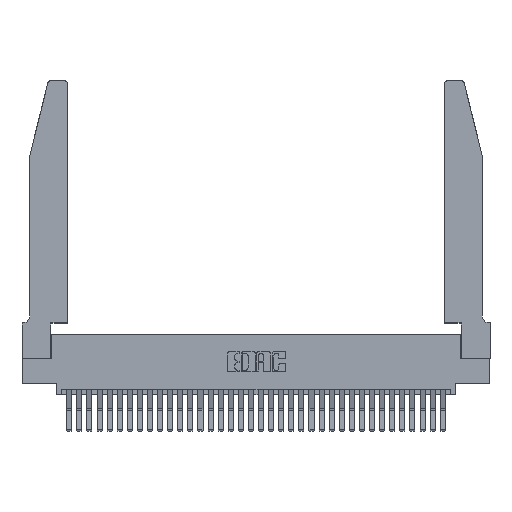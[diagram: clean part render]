
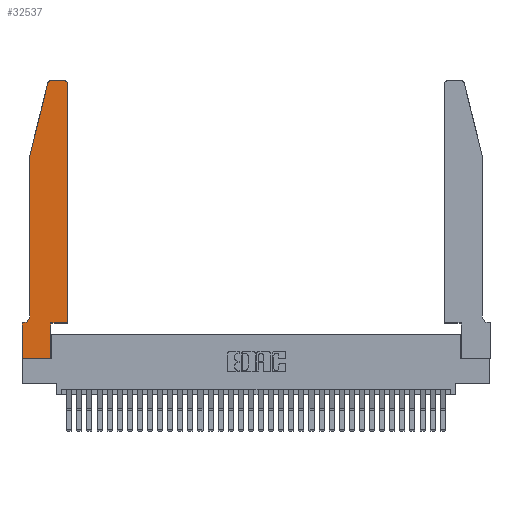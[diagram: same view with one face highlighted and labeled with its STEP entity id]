
A CAD part, top view. The second image highlights one B-rep face of the part: STEP entity #32537.
In plain terms, the highlighted planar face has unit normal (0, 0, 1).
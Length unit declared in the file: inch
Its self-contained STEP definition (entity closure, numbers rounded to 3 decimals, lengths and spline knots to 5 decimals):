
#457 = CARTESIAN_POINT ( 'NONE',  ( 0., 0.35, 0.37 ) ) ;
#463 = EDGE_CURVE ( 'NONE', #2228, #35208, #31307, .T. ) ;
#1337 = CARTESIAN_POINT ( 'NONE',  ( 0.0755, 0.42, 0.37 ) ) ;
#1734 = VECTOR ( 'NONE', #19854, 39.37008 ) ;
#1996 = DIRECTION ( 'NONE',  ( 1., 0., 0. ) ) ;
#2228 = VERTEX_POINT ( 'NONE', #1337 ) ;
#2260 = VERTEX_POINT ( 'NONE', #33999 ) ;
#2475 = CARTESIAN_POINT ( 'NONE',  ( 0.0755, 2., 0.37 ) ) ;
#2901 = CIRCLE ( 'NONE', #20183, 0.03 ) ;
#3153 = CARTESIAN_POINT ( 'NONE',  ( 0.2865, 0.35, 0.37 ) ) ;
#3363 = ORIENTED_EDGE ( 'NONE', *, *, #13857, .T. ) ;
#3400 = DIRECTION ( 'NONE',  ( 0., 0., 1. ) ) ;
#3839 = EDGE_CURVE ( 'NONE', #35208, #6836, #23939, .T. ) ;
#3932 = EDGE_CURVE ( 'NONE', #17710, #12336, #34092, .T. ) ;
#4143 = CARTESIAN_POINT ( 'NONE',  ( 0.0755, 2., 0.37 ) ) ;
#4219 = DIRECTION ( 'NONE',  ( 0., 0., -1. ) ) ;
#4291 = EDGE_CURVE ( 'NONE', #15877, #17710, #23027, .T. ) ;
#5108 = DIRECTION ( 'NONE',  ( -0.239, -0.971, 0. ) ) ;
#5288 = EDGE_CURVE ( 'NONE', #27021, #15877, #2901, .T. ) ;
#5319 = CARTESIAN_POINT ( 'NONE',  ( 0., 0., 0.37 ) ) ;
#5759 = ORIENTED_EDGE ( 'NONE', *, *, #23940, .T. ) ;
#5991 = LINE ( 'NONE', #10124, #12425 ) ;
#6008 = CARTESIAN_POINT ( 'NONE',  ( 0.2865, 0., 0.37 ) ) ;
#6277 = DIRECTION ( 'NONE',  ( 0., 0., 1. ) ) ;
#6380 = PLANE ( 'NONE',  #18262 ) ;
#6836 = VERTEX_POINT ( 'NONE', #22607 ) ;
#6881 = ORIENTED_EDGE ( 'NONE', *, *, #16343, .T. ) ;
#7226 = DIRECTION ( 'NONE',  ( 0., -1., 0. ) ) ;
#7690 = VECTOR ( 'NONE', #15726, 39.37008 ) ;
#7820 = LINE ( 'NONE', #2475, #23169 ) ;
#8686 = DIRECTION ( 'NONE',  ( 0., 1., 0. ) ) ;
#9730 = DIRECTION ( 'NONE',  ( -1., 0., 0. ) ) ;
#9872 = CARTESIAN_POINT ( 'NONE',  ( 0.4505, 0.35, 0.37 ) ) ;
#9953 = LINE ( 'NONE', #23705, #23200 ) ;
#10124 = CARTESIAN_POINT ( 'NONE',  ( 0.4505, 0.35, 0.37 ) ) ;
#11552 = ORIENTED_EDGE ( 'NONE', *, *, #14067, .T. ) ;
#11693 = EDGE_CURVE ( 'NONE', #35329, #2228, #9953, .T. ) ;
#11777 = CARTESIAN_POINT ( 'NONE',  ( 0.0055, 0.35, 0.37 ) ) ;
#12119 = CARTESIAN_POINT ( 'NONE',  ( 0.0055, 0.42, 0.37 ) ) ;
#12207 = VERTEX_POINT ( 'NONE', #27002 ) ;
#12327 = VERTEX_POINT ( 'NONE', #6008 ) ;
#12336 = VERTEX_POINT ( 'NONE', #17239 ) ;
#12425 = VECTOR ( 'NONE', #8686, 39.37008 ) ;
#13015 = FACE_OUTER_BOUND ( 'NONE', #28060, .T. ) ;
#13123 = EDGE_CURVE ( 'NONE', #12336, #35329, #7820, .T. ) ;
#13188 = LINE ( 'NONE', #9872, #19520 ) ;
#13271 = CARTESIAN_POINT ( 'NONE',  ( 0.284, 2.75, 0.37 ) ) ;
#13857 = EDGE_CURVE ( 'NONE', #12327, #12207, #21811, .T. ) ;
#14067 = EDGE_CURVE ( 'NONE', #2260, #27021, #5991, .T. ) ;
#14387 = LINE ( 'NONE', #30507, #18223 ) ;
#15726 = DIRECTION ( 'NONE',  ( -1., 0., 0. ) ) ;
#15877 = VERTEX_POINT ( 'NONE', #20146 ) ;
#16128 = ORIENTED_EDGE ( 'NONE', *, *, #26100, .T. ) ;
#16343 = EDGE_CURVE ( 'NONE', #27848, #12327, #14387, .T. ) ;
#16370 = ORIENTED_EDGE ( 'NONE', *, *, #5288, .T. ) ;
#16691 = AXIS2_PLACEMENT_3D ( 'NONE', #25144, #6277, #25493 ) ;
#17239 = CARTESIAN_POINT ( 'NONE',  ( 0.25487, 2.72718, 0.37 ) ) ;
#17710 = VERTEX_POINT ( 'NONE', #13271 ) ;
#18223 = VECTOR ( 'NONE', #24559, 39.37008 ) ;
#18262 = AXIS2_PLACEMENT_3D ( 'NONE', #457, #30561, #25472 ) ;
#19025 = AXIS2_PLACEMENT_3D ( 'NONE', #12119, #4219, #9730 ) ;
#19520 = VECTOR ( 'NONE', #1996, 39.37008 ) ;
#19854 = DIRECTION ( 'NONE',  ( 0., 1., 0. ) ) ;
#20038 = ORIENTED_EDGE ( 'NONE', *, *, #11693, .T. ) ;
#20146 = CARTESIAN_POINT ( 'NONE',  ( 0.4205, 2.75, 0.37 ) ) ;
#20183 = AXIS2_PLACEMENT_3D ( 'NONE', #32165, #3400, #28215 ) ;
#20365 = CARTESIAN_POINT ( 'NONE',  ( 0.0755, 0.35, 0.37 ) ) ;
#21811 = LINE ( 'NONE', #3153, #1734 ) ;
#22201 = VECTOR ( 'NONE', #28334, 39.37008 ) ;
#22607 = CARTESIAN_POINT ( 'NONE',  ( 0., 0.35, 0.37 ) ) ;
#23027 = LINE ( 'NONE', #26413, #7690 ) ;
#23169 = VECTOR ( 'NONE', #5108, 39.37008 ) ;
#23200 = VECTOR ( 'NONE', #7226, 39.37008 ) ;
#23705 = CARTESIAN_POINT ( 'NONE',  ( 0.0755, 2., 0.37 ) ) ;
#23939 = LINE ( 'NONE', #20365, #22201 ) ;
#23940 = EDGE_CURVE ( 'NONE', #12207, #2260, #13188, .T. ) ;
#23981 = ORIENTED_EDGE ( 'NONE', *, *, #13123, .T. ) ;
#24037 = CARTESIAN_POINT ( 'NONE',  ( 0.4505, 2.72, 0.37 ) ) ;
#24559 = DIRECTION ( 'NONE',  ( 1., 0., 0. ) ) ;
#24872 = DIRECTION ( 'NONE',  ( 0., -1., 0. ) ) ;
#25098 = ORIENTED_EDGE ( 'NONE', *, *, #3932, .T. ) ;
#25144 = CARTESIAN_POINT ( 'NONE',  ( 0.284, 2.72, 0.37 ) ) ;
#25469 = CARTESIAN_POINT ( 'NONE',  ( 0., 0., 0.37 ) ) ;
#25472 = DIRECTION ( 'NONE',  ( 1., 0., 0. ) ) ;
#25493 = DIRECTION ( 'NONE',  ( 1., 0., 0. ) ) ;
#25607 = ORIENTED_EDGE ( 'NONE', *, *, #3839, .T. ) ;
#26100 = EDGE_CURVE ( 'NONE', #6836, #27848, #32262, .T. ) ;
#26413 = CARTESIAN_POINT ( 'NONE',  ( 0.2605, 2.75, 0.37 ) ) ;
#27002 = CARTESIAN_POINT ( 'NONE',  ( 0.2865, 0.35, 0.37 ) ) ;
#27021 = VERTEX_POINT ( 'NONE', #24037 ) ;
#27848 = VERTEX_POINT ( 'NONE', #25469 ) ;
#28060 = EDGE_LOOP ( 'NONE', ( #28272, #25098, #23981, #20038, #32574, #25607, #16128, #6881, #3363, #5759, #11552, #16370 ) ) ;
#28215 = DIRECTION ( 'NONE',  ( 1., 0., 0. ) ) ;
#28272 = ORIENTED_EDGE ( 'NONE', *, *, #4291, .T. ) ;
#28334 = DIRECTION ( 'NONE',  ( -1., 0., 0. ) ) ;
#30507 = CARTESIAN_POINT ( 'NONE',  ( 0., 0., 0.37 ) ) ;
#30561 = DIRECTION ( 'NONE',  ( 0., 0., 1. ) ) ;
#31307 = CIRCLE ( 'NONE', #19025, 0.07 ) ;
#32165 = CARTESIAN_POINT ( 'NONE',  ( 0.4205, 2.72, 0.37 ) ) ;
#32262 = LINE ( 'NONE', #5319, #34392 ) ;
#32537 = ADVANCED_FACE ( 'NONE', ( #13015 ), #6380, .T. ) ;
#32574 = ORIENTED_EDGE ( 'NONE', *, *, #463, .T. ) ;
#33999 = CARTESIAN_POINT ( 'NONE',  ( 0.4505, 0.35, 0.37 ) ) ;
#34092 = CIRCLE ( 'NONE', #16691, 0.03 ) ;
#34392 = VECTOR ( 'NONE', #24872, 39.37008 ) ;
#35208 = VERTEX_POINT ( 'NONE', #11777 ) ;
#35329 = VERTEX_POINT ( 'NONE', #4143 ) ;
